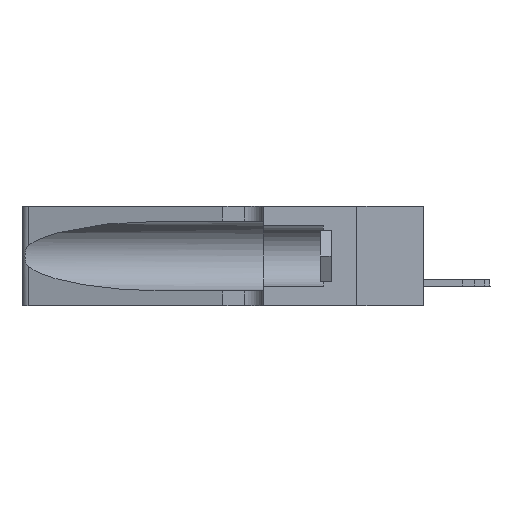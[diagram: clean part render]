
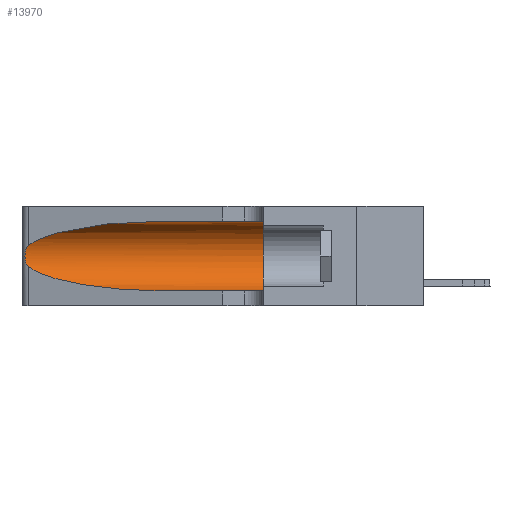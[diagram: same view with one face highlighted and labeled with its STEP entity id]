
A CAD part, left-side view. The second image highlights one B-rep face of the part: STEP entity #13970.
In plain terms, the highlighted cylindrical face has radius 3.308 mm (diameter 6.617 mm), a partial arc.
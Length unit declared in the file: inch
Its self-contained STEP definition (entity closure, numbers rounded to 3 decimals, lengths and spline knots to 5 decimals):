
#704 = DIRECTION ( 'NONE',  ( 0., 0., -1. ) ) ;
#1513 = CARTESIAN_POINT ( 'NONE',  ( 0.18966, 0.96281, 0.05475 ) ) ;
#2087 = EDGE_CURVE ( 'NONE', #27887, #32593, #20865, .T. ) ;
#3285 =( BOUNDED_CURVE ( )  B_SPLINE_CURVE ( 3, ( #12804, #28944, #1513, #9563 ),
 .UNSPECIFIED., .F., .T. ) 
 B_SPLINE_CURVE_WITH_KNOTS ( ( 4, 4 ),
 ( 3.44316, 4.71239 ),
 .UNSPECIFIED. ) 
 CURVE ( )  GEOMETRIC_REPRESENTATION_ITEM ( )  RATIONAL_B_SPLINE_CURVE ( ( 1., 0.87, 0.87, 1. ) ) 
 REPRESENTATION_ITEM ( '' )  );
#3735 = CARTESIAN_POINT ( 'NONE',  ( 0.25789, 1.23486, 0.15765 ) ) ;
#4402 =( BOUNDED_CURVE ( )  B_SPLINE_CURVE ( 3, ( #7824, #4951, #32521, #21458 ),
 .UNSPECIFIED., .F., .F. ) 
 B_SPLINE_CURVE_WITH_KNOTS ( ( 4, 4 ),
 ( 1.5708, 2.84003 ),
 .UNSPECIFIED. ) 
 CURVE ( )  GEOMETRIC_REPRESENTATION_ITEM ( )  RATIONAL_B_SPLINE_CURVE ( ( 1., 0.87, 0.87, 1. ) ) 
 REPRESENTATION_ITEM ( '' )  );
#4919 = VERTEX_POINT ( 'NONE', #7104 ) ;
#4951 = CARTESIAN_POINT ( 'NONE',  ( 0.18966, 0.96281, 0.31525 ) ) ;
#6261 = CARTESIAN_POINT ( 'NONE',  ( 0.25487, 1.22718, 0.22369 ) ) ;
#6659 = VERTEX_POINT ( 'NONE', #14632 ) ;
#6711 = CARTESIAN_POINT ( 'NONE',  ( 0.25487, 1.22718, 0.14631 ) ) ;
#7104 = CARTESIAN_POINT ( 'NONE',  ( 0.1305, 0.35, 0.05475 ) ) ;
#7824 = CARTESIAN_POINT ( 'NONE',  ( 0.1305, 0.72297, 0.31525 ) ) ;
#8107 = ORIENTED_EDGE ( 'NONE', *, *, #29117, .T. ) ;
#8502 = VECTOR ( 'NONE', #14227, 39.37008 ) ;
#8774 = CARTESIAN_POINT ( 'NONE',  ( 0.1305, 1.61858, 0.185 ) ) ;
#9205 = AXIS2_PLACEMENT_3D ( 'NONE', #29580, #18931, #18811 ) ;
#9307 = DIRECTION ( 'NONE',  ( 0., -1., 0. ) ) ;
#9379 = CARTESIAN_POINT ( 'NONE',  ( 0.25787, 1.23484, 0.2124 ) ) ;
#9563 = CARTESIAN_POINT ( 'NONE',  ( 0.1305, 0.72297, 0.05475 ) ) ;
#11163 = EDGE_CURVE ( 'NONE', #11455, #4919, #27350, .T. ) ;
#11455 = VERTEX_POINT ( 'NONE', #30370 ) ;
#12153 = CARTESIAN_POINT ( 'NONE',  ( 0.26075, 1.23896, 0.19203 ) ) ;
#12347 = LINE ( 'NONE', #31365, #31635 ) ;
#12804 = CARTESIAN_POINT ( 'NONE',  ( 0.25487, 1.22718, 0.14631 ) ) ;
#13970 = ADVANCED_FACE ( 'NONE', ( #24017 ), #31366, .F. ) ;
#14227 = DIRECTION ( 'NONE',  ( 0., -1., 0. ) ) ;
#14245 = CARTESIAN_POINT ( 'NONE',  ( 0.1305, 0.72297, 0.05475 ) ) ;
#14310 = DIRECTION ( 'NONE',  ( 0., -1., 0. ) ) ;
#14632 = CARTESIAN_POINT ( 'NONE',  ( 0.1305, 0.72297, 0.31525 ) ) ;
#14906 = CARTESIAN_POINT ( 'NONE',  ( 0.25555, 1.22993, 0.14849 ) ) ;
#15806 = LINE ( 'NONE', #33609, #8502 ) ;
#17172 = CARTESIAN_POINT ( 'NONE',  ( 0.26017, 1.23833, 0.17102 ) ) ;
#18811 = DIRECTION ( 'NONE',  ( 0., 0., 1. ) ) ;
#18931 = DIRECTION ( 'NONE',  ( 0., 1., 0. ) ) ;
#19175 = ORIENTED_EDGE ( 'NONE', *, *, #11163, .F. ) ;
#20166 = CARTESIAN_POINT ( 'NONE',  ( 0.26018, 1.23835, 0.19895 ) ) ;
#20193 = AXIS2_PLACEMENT_3D ( 'NONE', #8774, #14310, #704 ) ;
#20272 = VERTEX_POINT ( 'NONE', #14245 ) ;
#20865 = B_SPLINE_CURVE_WITH_KNOTS ( 'NONE', 3,
 ( #6261, #34033, #22748, #9379, #28523, #20166, #12153, #31313, #17172, #25384, #3735, #33699, #14906, #22859 ),
 .UNSPECIFIED., .F., .F.,
 ( 4, 2, 2, 2, 2, 2, 4 ),
 ( 0., 0.00027, 0.00053, 0.00107, 0.0016, 0.00187, 0.00214 ),
 .UNSPECIFIED. ) ;
#21458 = CARTESIAN_POINT ( 'NONE',  ( 0.25487, 1.22718, 0.22369 ) ) ;
#21800 = EDGE_LOOP ( 'NONE', ( #29624, #23170, #29618, #8107, #19175, #22214 ) ) ;
#22214 = ORIENTED_EDGE ( 'NONE', *, *, #25682, .F. ) ;
#22748 = CARTESIAN_POINT ( 'NONE',  ( 0.25639, 1.23184, 0.21858 ) ) ;
#22859 = CARTESIAN_POINT ( 'NONE',  ( 0.25487, 1.22718, 0.14631 ) ) ;
#23170 = ORIENTED_EDGE ( 'NONE', *, *, #2087, .T. ) ;
#24017 = FACE_OUTER_BOUND ( 'NONE', #21800, .T. ) ;
#24789 = CARTESIAN_POINT ( 'NONE',  ( 0.25487, 1.22718, 0.22369 ) ) ;
#25384 = CARTESIAN_POINT ( 'NONE',  ( 0.25856, 1.23593, 0.16098 ) ) ;
#25682 = EDGE_CURVE ( 'NONE', #6659, #11455, #12347, .T. ) ;
#26589 = EDGE_CURVE ( 'NONE', #6659, #27887, #4402, .T. ) ;
#27350 = CIRCLE ( 'NONE', #9205, 0.13025 ) ;
#27887 = VERTEX_POINT ( 'NONE', #24789 ) ;
#28523 = CARTESIAN_POINT ( 'NONE',  ( 0.25854, 1.2359, 0.20912 ) ) ;
#28944 = CARTESIAN_POINT ( 'NONE',  ( 0.2373, 1.15595, 0.08982 ) ) ;
#29117 = EDGE_CURVE ( 'NONE', #20272, #4919, #15806, .T. ) ;
#29580 = CARTESIAN_POINT ( 'NONE',  ( 0.1305, 0.35, 0.185 ) ) ;
#29618 = ORIENTED_EDGE ( 'NONE', *, *, #32889, .T. ) ;
#29624 = ORIENTED_EDGE ( 'NONE', *, *, #26589, .T. ) ;
#30370 = CARTESIAN_POINT ( 'NONE',  ( 0.1305, 0.35, 0.31525 ) ) ;
#31313 = CARTESIAN_POINT ( 'NONE',  ( 0.26075, 1.23896, 0.178 ) ) ;
#31365 = CARTESIAN_POINT ( 'NONE',  ( 0.1305, 1.61858, 0.31525 ) ) ;
#31366 = CYLINDRICAL_SURFACE ( 'NONE', #20193, 0.13025 ) ;
#31635 = VECTOR ( 'NONE', #9307, 39.37008 ) ;
#32521 = CARTESIAN_POINT ( 'NONE',  ( 0.2373, 1.15595, 0.28018 ) ) ;
#32593 = VERTEX_POINT ( 'NONE', #6711 ) ;
#32889 = EDGE_CURVE ( 'NONE', #32593, #20272, #3285, .T. ) ;
#33609 = CARTESIAN_POINT ( 'NONE',  ( 0.1305, 1.61858, 0.05475 ) ) ;
#33699 = CARTESIAN_POINT ( 'NONE',  ( 0.25639, 1.23186, 0.15144 ) ) ;
#34033 = CARTESIAN_POINT ( 'NONE',  ( 0.25555, 1.22994, 0.2215 ) ) ;
